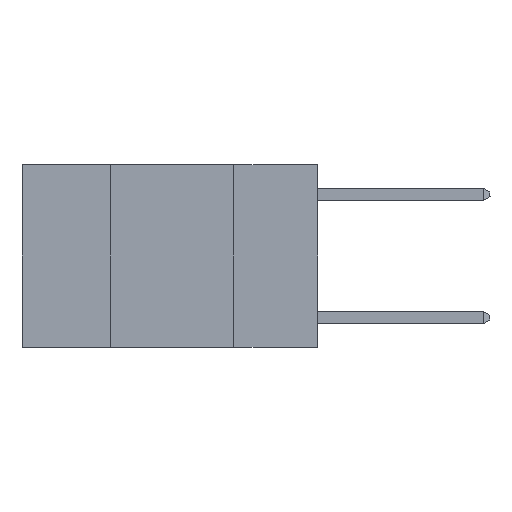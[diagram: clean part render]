
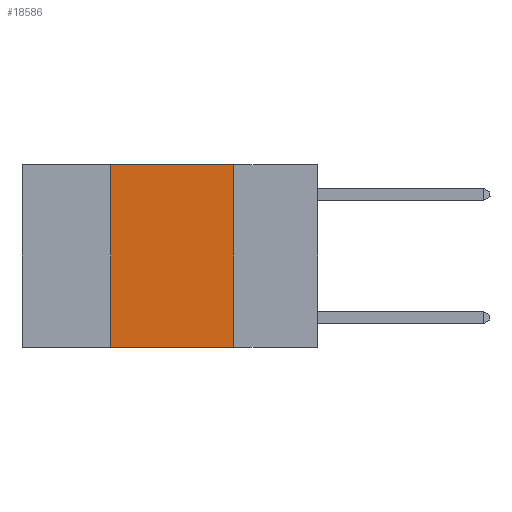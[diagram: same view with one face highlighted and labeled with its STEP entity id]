
A CAD part, left-side view. The second image highlights one B-rep face of the part: STEP entity #18586.
In plain terms, the highlighted planar face has unit normal (-1, 0, 0).
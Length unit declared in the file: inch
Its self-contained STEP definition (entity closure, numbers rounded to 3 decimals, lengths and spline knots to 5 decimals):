
#9 = LINE ( 'NONE', #9658, #24176 ) ;
#536 = CARTESIAN_POINT ( 'NONE',  ( 0., 0.42, 0. ) ) ;
#1723 = CARTESIAN_POINT ( 'NONE',  ( 0., 0.42, -0.37 ) ) ;
#2132 = LINE ( 'NONE', #13522, #14783 ) ;
#3935 = VERTEX_POINT ( 'NONE', #536 ) ;
#4599 = ORIENTED_EDGE ( 'NONE', *, *, #26801, .F. ) ;
#5066 = LINE ( 'NONE', #22861, #11639 ) ;
#6425 = EDGE_LOOP ( 'NONE', ( #9609, #4599, #25543, #14481 ) ) ;
#6562 = DIRECTION ( 'NONE',  ( 0., 0., -1. ) ) ;
#7834 = VERTEX_POINT ( 'NONE', #1723 ) ;
#9597 = VERTEX_POINT ( 'NONE', #31052 ) ;
#9609 = ORIENTED_EDGE ( 'NONE', *, *, #13870, .F. ) ;
#9658 = CARTESIAN_POINT ( 'NONE',  ( 0., 0.6, 0. ) ) ;
#11463 = CARTESIAN_POINT ( 'NONE',  ( 0., 0.6, 0. ) ) ;
#11639 = VECTOR ( 'NONE', #30255, 39.37008 ) ;
#13522 = CARTESIAN_POINT ( 'NONE',  ( 0., 0.17, 0. ) ) ;
#13814 = DIRECTION ( 'NONE',  ( 0., 0., -1. ) ) ;
#13870 = EDGE_CURVE ( 'NONE', #9597, #23693, #2132, .T. ) ;
#13949 = EDGE_CURVE ( 'NONE', #7834, #23693, #19172, .T. ) ;
#14379 = AXIS2_PLACEMENT_3D ( 'NONE', #11463, #26215, #13814 ) ;
#14481 = ORIENTED_EDGE ( 'NONE', *, *, #13949, .T. ) ;
#14783 = VECTOR ( 'NONE', #6562, 39.37008 ) ;
#14911 = DIRECTION ( 'NONE',  ( 0., -1., 0. ) ) ;
#16644 = PLANE ( 'NONE',  #14379 ) ;
#18586 = ADVANCED_FACE ( 'NONE', ( #19018 ), #16644, .F. ) ;
#19018 = FACE_OUTER_BOUND ( 'NONE', #6425, .T. ) ;
#19061 = CARTESIAN_POINT ( 'NONE',  ( 0., 0.17, -0.37 ) ) ;
#19172 = LINE ( 'NONE', #23872, #29852 ) ;
#22861 = CARTESIAN_POINT ( 'NONE',  ( 0., 0.42, 0. ) ) ;
#23693 = VERTEX_POINT ( 'NONE', #19061 ) ;
#23872 = CARTESIAN_POINT ( 'NONE',  ( 0., 0.6, -0.37 ) ) ;
#24176 = VECTOR ( 'NONE', #28861, 39.37008 ) ;
#25543 = ORIENTED_EDGE ( 'NONE', *, *, #29575, .F. ) ;
#26215 = DIRECTION ( 'NONE',  ( 1., 0., 0. ) ) ;
#26801 = EDGE_CURVE ( 'NONE', #3935, #9597, #9, .T. ) ;
#28861 = DIRECTION ( 'NONE',  ( 0., -1., 0. ) ) ;
#29575 = EDGE_CURVE ( 'NONE', #7834, #3935, #5066, .T. ) ;
#29852 = VECTOR ( 'NONE', #14911, 39.37008 ) ;
#30255 = DIRECTION ( 'NONE',  ( 0., 0., 1. ) ) ;
#31052 = CARTESIAN_POINT ( 'NONE',  ( 0., 0.17, 0. ) ) ;
